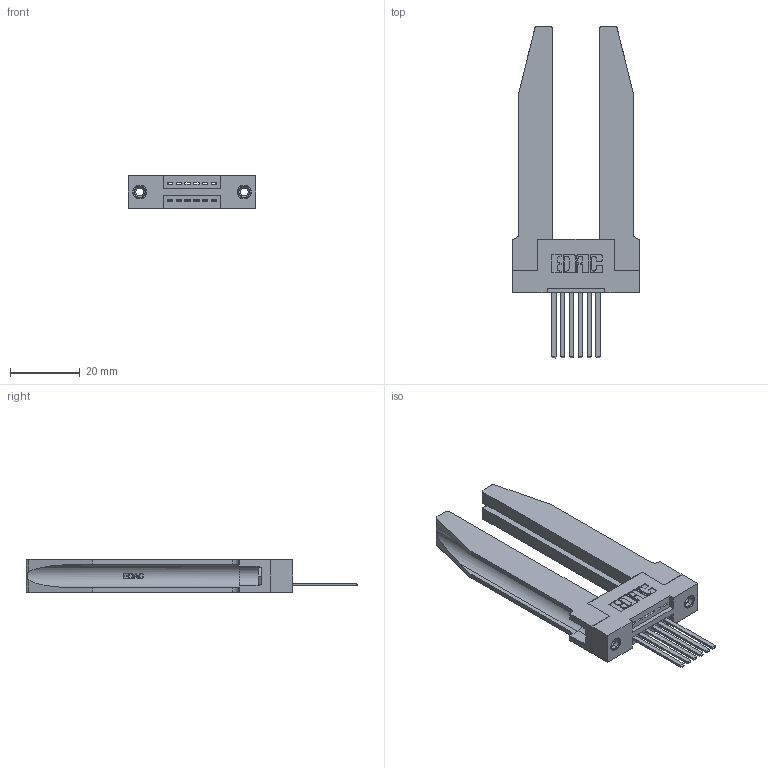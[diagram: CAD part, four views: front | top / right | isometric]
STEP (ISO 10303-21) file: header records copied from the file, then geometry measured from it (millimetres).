
FILE_DESCRIPTION (( 'STEP AP203' ), '1' );
FILE_NAME ('345-006-544-178.STEP', '2019-10-03T16:13:11', ( '' ), ( '' ), 'SwSTEP 2.0', 'SolidWorks 2016', '' );
FILE_SCHEMA (( 'CONFIG_CONTROL_DESIGN' ));
Length unit declared in the file: inch
Products named in the file (5): 345-250-001_345-250-001-102; 345-220-078_345-220-078; 345-292-001_345-293-144; 345-006-544-178; 345 Part_Flush Mounting Lugs - 0.156 Dia-TH
Assembly tree (11 placements, depth 2):
  345-006-544-178
    345 Part_Flush Mounting Lugs - 0.156 Dia-TH
    345-292-001_345-293-144  x6
    345-250-001_345-250-001-102  x2
    345-220-078_345-220-078  x2
Bounding box: 36.47 x 94.92 x 9.4 mm (x, y, z)
Volume: 11009.4 mm3; surface area: 10869.2 mm2
Topology: 11 solids, 11 shells, 672 faces, 1897 edges, 1246 vertices
Faces by surface type: plane 438, cylinder 182, bspline 36, cone 12, torus 4
Entity records: 13918 total; most frequent: CARTESIAN_POINT 3309, ORIENTED_EDGE 2146, DIRECTION 1947, EDGE_CURVE 1073, VECTOR 827, LINE 827, VERTEX_POINT 708, AXIS2_PLACEMENT_3D 560
